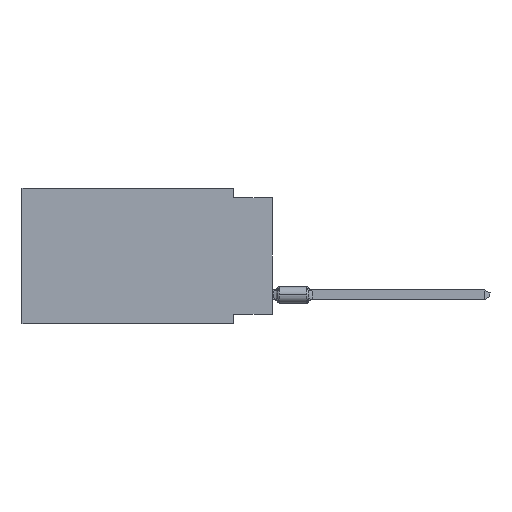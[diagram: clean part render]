
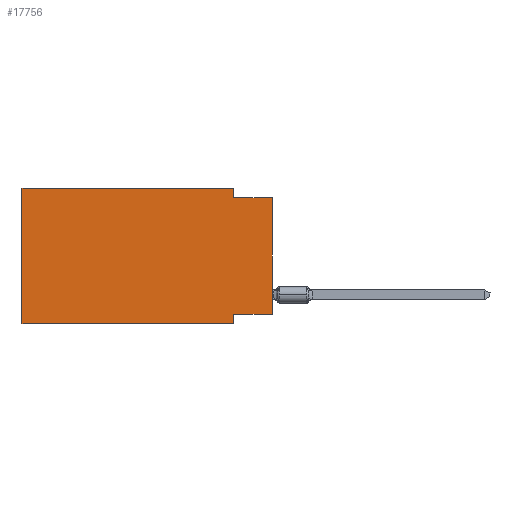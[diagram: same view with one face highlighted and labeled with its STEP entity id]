
A CAD part, left-side view. The second image highlights one B-rep face of the part: STEP entity #17756.
In plain terms, the highlighted planar face has unit normal (-1, 0, 0).
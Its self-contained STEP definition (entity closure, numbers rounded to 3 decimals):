
#152 = EDGE_CURVE ( 'NONE', #23496, #7851, #23091, .T. ) ;
#156 = EDGE_CURVE ( 'NONE', #17947, #34404, #6931, .T. ) ;
#286 = VECTOR ( 'NONE', #14582, 1000. ) ;
#635 = CARTESIAN_POINT ( 'NONE',  ( 0., 0., -0.635 ) ) ;
#1400 = ORIENTED_EDGE ( 'NONE', *, *, #152, .T. ) ;
#2266 = EDGE_LOOP ( 'NONE', ( #33251, #41212, #2768, #16265, #26541, #1400, #12985, #6381 ) ) ;
#2768 = ORIENTED_EDGE ( 'NONE', *, *, #12870, .F. ) ;
#3657 = CARTESIAN_POINT ( 'NONE',  ( 0., 0., -8.255 ) ) ;
#3838 = LINE ( 'NONE', #635, #15206 ) ;
#3957 = CARTESIAN_POINT ( 'NONE',  ( 0., 16.383, 0. ) ) ;
#4691 = DIRECTION ( 'NONE',  ( 0., 0., -1. ) ) ;
#5257 = CARTESIAN_POINT ( 'NONE',  ( 0., 2.54, 0. ) ) ;
#5665 = CARTESIAN_POINT ( 'NONE',  ( 0., 0., -8.255 ) ) ;
#6381 = ORIENTED_EDGE ( 'NONE', *, *, #8707, .F. ) ;
#6931 = LINE ( 'NONE', #35267, #22954 ) ;
#7572 = CARTESIAN_POINT ( 'NONE',  ( 0., 0., -0.635 ) ) ;
#7851 = VERTEX_POINT ( 'NONE', #41374 ) ;
#8707 = EDGE_CURVE ( 'NONE', #17947, #14741, #18439, .T. ) ;
#9903 = LINE ( 'NONE', #22877, #286 ) ;
#10848 = VERTEX_POINT ( 'NONE', #18679 ) ;
#12337 = CARTESIAN_POINT ( 'NONE',  ( 0., 16.383, 0. ) ) ;
#12758 = DIRECTION ( 'NONE',  ( 0., -1., 0. ) ) ;
#12870 = EDGE_CURVE ( 'NONE', #20835, #27253, #37074, .T. ) ;
#12985 = ORIENTED_EDGE ( 'NONE', *, *, #38389, .F. ) ;
#14582 = DIRECTION ( 'NONE',  ( 0., 0., 1. ) ) ;
#14741 = VERTEX_POINT ( 'NONE', #29548 ) ;
#15206 = VECTOR ( 'NONE', #33215, 1000. ) ;
#16265 = ORIENTED_EDGE ( 'NONE', *, *, #21629, .F. ) ;
#16945 = DIRECTION ( 'NONE',  ( 1., 0., 0. ) ) ;
#17756 = ADVANCED_FACE ( 'NONE', ( #39502 ), #23731, .F. ) ;
#17947 = VERTEX_POINT ( 'NONE', #3657 ) ;
#18439 = LINE ( 'NONE', #5665, #20092 ) ;
#18679 = CARTESIAN_POINT ( 'NONE',  ( 0., 16.383, 0. ) ) ;
#19071 = VECTOR ( 'NONE', #4691, 1000. ) ;
#19698 = DIRECTION ( 'NONE',  ( 0., -1., 0. ) ) ;
#20092 = VECTOR ( 'NONE', #28228, 1000. ) ;
#20835 = VERTEX_POINT ( 'NONE', #5257 ) ;
#20870 = CARTESIAN_POINT ( 'NONE',  ( 0., 2.54, 0. ) ) ;
#21599 = VECTOR ( 'NONE', #19698, 1000. ) ;
#21629 = EDGE_CURVE ( 'NONE', #10848, #20835, #31510, .T. ) ;
#22877 = CARTESIAN_POINT ( 'NONE',  ( 0., 16.383, 0. ) ) ;
#22954 = VECTOR ( 'NONE', #35475, 1000. ) ;
#23091 = LINE ( 'NONE', #26506, #21599 ) ;
#23496 = VERTEX_POINT ( 'NONE', #27944 ) ;
#23731 = PLANE ( 'NONE',  #42040 ) ;
#25120 = LINE ( 'NONE', #33153, #40350 ) ;
#26454 = CARTESIAN_POINT ( 'NONE',  ( 0., 2.54, -0.635 ) ) ;
#26506 = CARTESIAN_POINT ( 'NONE',  ( 0., 16.383, -8.89 ) ) ;
#26541 = ORIENTED_EDGE ( 'NONE', *, *, #38848, .F. ) ;
#27253 = VERTEX_POINT ( 'NONE', #26454 ) ;
#27944 = CARTESIAN_POINT ( 'NONE',  ( 0., 16.383, -8.89 ) ) ;
#28228 = DIRECTION ( 'NONE',  ( 0., 1., 0. ) ) ;
#29548 = CARTESIAN_POINT ( 'NONE',  ( 0., 2.54, -8.255 ) ) ;
#29928 = DIRECTION ( 'NONE',  ( 0., 0., -1. ) ) ;
#29948 = DIRECTION ( 'NONE',  ( 0., 0., -1. ) ) ;
#30440 = VECTOR ( 'NONE', #12758, 1000. ) ;
#30829 = EDGE_CURVE ( 'NONE', #27253, #34404, #3838, .T. ) ;
#31510 = LINE ( 'NONE', #12337, #30440 ) ;
#33153 = CARTESIAN_POINT ( 'NONE',  ( 0., 2.54, -8.89 ) ) ;
#33215 = DIRECTION ( 'NONE',  ( 0., -1., 0. ) ) ;
#33251 = ORIENTED_EDGE ( 'NONE', *, *, #156, .T. ) ;
#34404 = VERTEX_POINT ( 'NONE', #7572 ) ;
#35267 = CARTESIAN_POINT ( 'NONE',  ( 0., 0., 0. ) ) ;
#35475 = DIRECTION ( 'NONE',  ( 0., 0., 1. ) ) ;
#37074 = LINE ( 'NONE', #20870, #19071 ) ;
#38389 = EDGE_CURVE ( 'NONE', #14741, #7851, #25120, .T. ) ;
#38848 = EDGE_CURVE ( 'NONE', #23496, #10848, #9903, .T. ) ;
#39502 = FACE_OUTER_BOUND ( 'NONE', #2266, .T. ) ;
#40350 = VECTOR ( 'NONE', #29948, 1000. ) ;
#41212 = ORIENTED_EDGE ( 'NONE', *, *, #30829, .F. ) ;
#41374 = CARTESIAN_POINT ( 'NONE',  ( 0., 2.54, -8.89 ) ) ;
#42040 = AXIS2_PLACEMENT_3D ( 'NONE', #3957, #16945, #29928 ) ;
